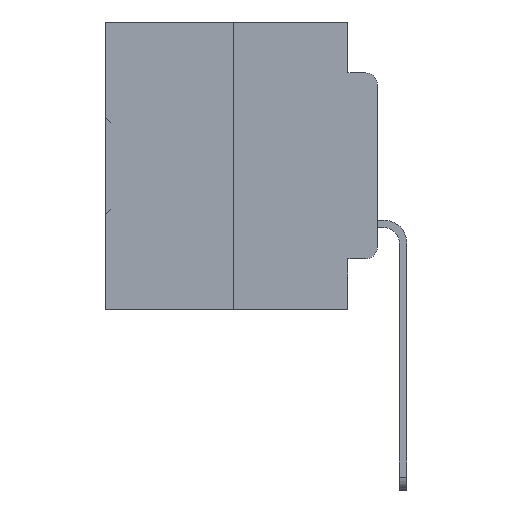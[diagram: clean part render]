
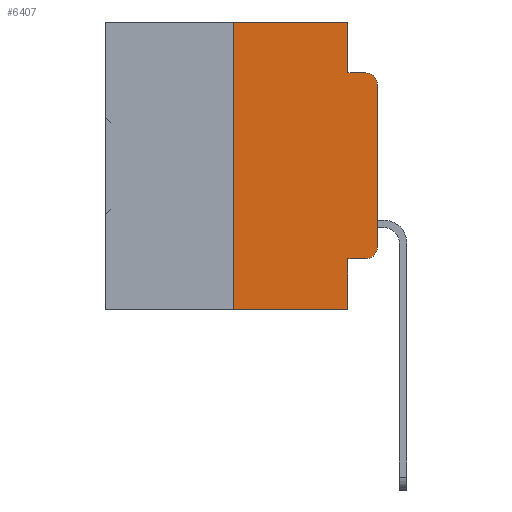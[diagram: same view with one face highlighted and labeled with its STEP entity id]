
A CAD part, left-side view. The second image highlights one B-rep face of the part: STEP entity #6407.
In plain terms, the highlighted planar face has unit normal (-1, 0, 0).
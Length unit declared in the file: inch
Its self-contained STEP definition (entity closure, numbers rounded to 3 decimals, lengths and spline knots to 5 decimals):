
#642 = CARTESIAN_POINT ( 'NONE',  ( 0., 0.051, -0.4115 ) ) ;
#1075 = ORIENTED_EDGE ( 'NONE', *, *, #34210, .T. ) ;
#1217 = VECTOR ( 'NONE', #3121, 39.37008 ) ;
#1562 = DIRECTION ( 'NONE',  ( 0., -1., 0. ) ) ;
#1948 = CARTESIAN_POINT ( 'NONE',  ( 0., 0.25, -0.5 ) ) ;
#2539 = DIRECTION ( 'NONE',  ( 0., 0., 1. ) ) ;
#2823 = VERTEX_POINT ( 'NONE', #35240 ) ;
#3121 = DIRECTION ( 'NONE',  ( 0., 0., -1. ) ) ;
#3204 = ORIENTED_EDGE ( 'NONE', *, *, #6514, .T. ) ;
#3464 = VERTEX_POINT ( 'NONE', #17280 ) ;
#3637 = LINE ( 'NONE', #17508, #11650 ) ;
#3780 = CARTESIAN_POINT ( 'NONE',  ( 0., 0.051, -0.4115 ) ) ;
#4108 = VERTEX_POINT ( 'NONE', #1948 ) ;
#4972 = CARTESIAN_POINT ( 'NONE',  ( 0., 0.02, -0.3915 ) ) ;
#5248 = VERTEX_POINT ( 'NONE', #37651 ) ;
#5429 = CARTESIAN_POINT ( 'NONE',  ( 0., 0.25, 0. ) ) ;
#6111 = ORIENTED_EDGE ( 'NONE', *, *, #34923, .F. ) ;
#6407 = ADVANCED_FACE ( 'NONE', ( #27651 ), #25613, .F. ) ;
#6514 = EDGE_CURVE ( 'NONE', #2823, #17156, #16790, .T. ) ;
#6760 = EDGE_CURVE ( 'NONE', #37214, #37954, #31351, .T. ) ;
#6975 = VECTOR ( 'NONE', #1562, 39.37008 ) ;
#7918 = LINE ( 'NONE', #25715, #6975 ) ;
#8030 = DIRECTION ( 'NONE',  ( 0., 0., -1. ) ) ;
#9309 = VECTOR ( 'NONE', #19053, 39.37008 ) ;
#9361 = CARTESIAN_POINT ( 'NONE',  ( 0., 0.02, -0.0885 ) ) ;
#9923 = ORIENTED_EDGE ( 'NONE', *, *, #37077, .T. ) ;
#10568 = CARTESIAN_POINT ( 'NONE',  ( 0., 0.473, 0. ) ) ;
#11650 = VECTOR ( 'NONE', #38315, 39.37008 ) ;
#12239 = EDGE_CURVE ( 'NONE', #18566, #37214, #7918, .T. ) ;
#12895 = ORIENTED_EDGE ( 'NONE', *, *, #20930, .F. ) ;
#13564 = DIRECTION ( 'NONE',  ( 0., 0., -1. ) ) ;
#13886 = LINE ( 'NONE', #31603, #38597 ) ;
#14377 = CARTESIAN_POINT ( 'NONE',  ( 0., 0.051, 0. ) ) ;
#14411 = AXIS2_PLACEMENT_3D ( 'NONE', #32660, #14701, #35629 ) ;
#14701 = DIRECTION ( 'NONE',  ( -1., 0., 0. ) ) ;
#15648 = CARTESIAN_POINT ( 'NONE',  ( 0., 0.051, -0.0885 ) ) ;
#15982 = VECTOR ( 'NONE', #31860, 39.37008 ) ;
#16007 = EDGE_CURVE ( 'NONE', #4108, #3464, #34181, .T. ) ;
#16790 = CIRCLE ( 'NONE', #33948, 0.02 ) ;
#17156 = VERTEX_POINT ( 'NONE', #19413 ) ;
#17280 = CARTESIAN_POINT ( 'NONE',  ( 0., 0.051, -0.5 ) ) ;
#17483 = ORIENTED_EDGE ( 'NONE', *, *, #26455, .T. ) ;
#17508 = CARTESIAN_POINT ( 'NONE',  ( 0., 0.051, -0.0885 ) ) ;
#18163 = CARTESIAN_POINT ( 'NONE',  ( 0., 0.051, 0. ) ) ;
#18546 = ORIENTED_EDGE ( 'NONE', *, *, #12239, .F. ) ;
#18566 = VERTEX_POINT ( 'NONE', #5429 ) ;
#19053 = DIRECTION ( 'NONE',  ( 0., -1., 0. ) ) ;
#19413 = CARTESIAN_POINT ( 'NONE',  ( 0., 0., -0.3915 ) ) ;
#20930 = EDGE_CURVE ( 'NONE', #4108, #18566, #38785, .T. ) ;
#21180 = VECTOR ( 'NONE', #2539, 39.37008 ) ;
#22525 = ORIENTED_EDGE ( 'NONE', *, *, #35645, .F. ) ;
#22725 = DIRECTION ( 'NONE',  ( 0., 0., 1. ) ) ;
#24042 = LINE ( 'NONE', #28899, #15982 ) ;
#25613 = PLANE ( 'NONE',  #31947 ) ;
#25715 = CARTESIAN_POINT ( 'NONE',  ( 0., 0.473, 0. ) ) ;
#25801 = CIRCLE ( 'NONE', #14411, 0.02 ) ;
#26073 = VERTEX_POINT ( 'NONE', #642 ) ;
#26109 = DIRECTION ( 'NONE',  ( -1., 0., 0. ) ) ;
#26359 = ORIENTED_EDGE ( 'NONE', *, *, #6760, .F. ) ;
#26455 = EDGE_CURVE ( 'NONE', #5248, #34096, #25801, .T. ) ;
#26830 = LINE ( 'NONE', #3780, #35623 ) ;
#27651 = FACE_OUTER_BOUND ( 'NONE', #35809, .T. ) ;
#28899 = CARTESIAN_POINT ( 'NONE',  ( 0., 0.051, 0. ) ) ;
#28922 = ORIENTED_EDGE ( 'NONE', *, *, #16007, .T. ) ;
#31351 = LINE ( 'NONE', #18163, #1217 ) ;
#31563 = DIRECTION ( 'NONE',  ( 1., 0., 0. ) ) ;
#31603 = CARTESIAN_POINT ( 'NONE',  ( 0., 0., 0. ) ) ;
#31860 = DIRECTION ( 'NONE',  ( 0., 0., -1. ) ) ;
#31947 = AXIS2_PLACEMENT_3D ( 'NONE', #10568, #31563, #13564 ) ;
#32660 = CARTESIAN_POINT ( 'NONE',  ( 0., 0.02, -0.1085 ) ) ;
#33872 = DIRECTION ( 'NONE',  ( 0., -1., 0. ) ) ;
#33948 = AXIS2_PLACEMENT_3D ( 'NONE', #4972, #26109, #8030 ) ;
#34096 = VERTEX_POINT ( 'NONE', #9361 ) ;
#34181 = LINE ( 'NONE', #36858, #9309 ) ;
#34210 = EDGE_CURVE ( 'NONE', #26073, #2823, #26830, .T. ) ;
#34923 = EDGE_CURVE ( 'NONE', #26073, #3464, #24042, .T. ) ;
#35240 = CARTESIAN_POINT ( 'NONE',  ( 0., 0.02, -0.4115 ) ) ;
#35623 = VECTOR ( 'NONE', #33872, 39.37008 ) ;
#35629 = DIRECTION ( 'NONE',  ( 0., 0., -1. ) ) ;
#35645 = EDGE_CURVE ( 'NONE', #37954, #34096, #3637, .T. ) ;
#35809 = EDGE_LOOP ( 'NONE', ( #9923, #17483, #22525, #26359, #18546, #12895, #28922, #6111, #1075, #3204 ) ) ;
#36858 = CARTESIAN_POINT ( 'NONE',  ( 0., 0.473, -0.5 ) ) ;
#37077 = EDGE_CURVE ( 'NONE', #17156, #5248, #13886, .T. ) ;
#37214 = VERTEX_POINT ( 'NONE', #14377 ) ;
#37651 = CARTESIAN_POINT ( 'NONE',  ( 0., 0., -0.1085 ) ) ;
#37954 = VERTEX_POINT ( 'NONE', #15648 ) ;
#38315 = DIRECTION ( 'NONE',  ( 0., -1., 0. ) ) ;
#38492 = CARTESIAN_POINT ( 'NONE',  ( 0., 0.25, 0. ) ) ;
#38597 = VECTOR ( 'NONE', #22725, 39.37008 ) ;
#38785 = LINE ( 'NONE', #38492, #21180 ) ;
